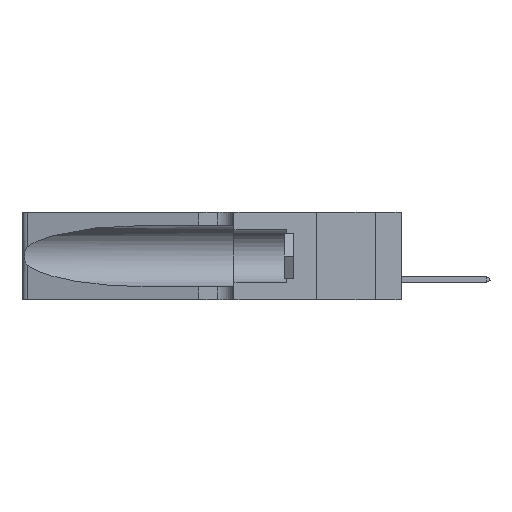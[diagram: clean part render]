
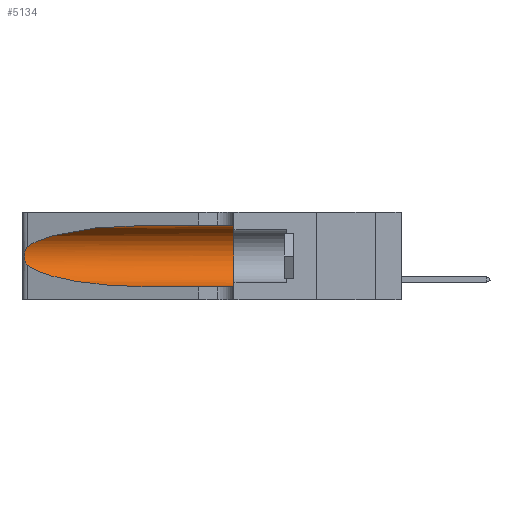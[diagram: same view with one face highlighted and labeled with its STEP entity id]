
A CAD part, left-side view. The second image highlights one B-rep face of the part: STEP entity #5134.
In plain terms, the highlighted cylindrical face has radius 3.308 mm (diameter 6.617 mm), a partial arc.
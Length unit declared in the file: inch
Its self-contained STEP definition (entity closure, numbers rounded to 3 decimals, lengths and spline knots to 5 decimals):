
#425 = AXIS2_PLACEMENT_3D ( 'NONE', #13948, #22495, #15842 ) ;
#451 = CARTESIAN_POINT ( 'NONE',  ( 0.25555, 1.22993, 0.14849 ) ) ;
#1627 = CARTESIAN_POINT ( 'NONE',  ( 0.25487, 1.22718, 0.22369 ) ) ;
#2332 = EDGE_CURVE ( 'NONE', #14540, #21522, #24726, .T. ) ;
#2381 =( BOUNDED_CURVE ( )  B_SPLINE_CURVE ( 3, ( #17505, #17337, #19689, #6827 ),
 .UNSPECIFIED., .F., .F. ) 
 B_SPLINE_CURVE_WITH_KNOTS ( ( 4, 4 ),
 ( 3.44316, 4.71239 ),
 .UNSPECIFIED. ) 
 CURVE ( )  GEOMETRIC_REPRESENTATION_ITEM ( )  RATIONAL_B_SPLINE_CURVE ( ( 1., 0.87, 0.87, 1. ) ) 
 REPRESENTATION_ITEM ( '' )  );
#2425 = ORIENTED_EDGE ( 'NONE', *, *, #22101, .T. ) ;
#2613 = CARTESIAN_POINT ( 'NONE',  ( 0.25639, 1.23184, 0.21858 ) ) ;
#3595 = CARTESIAN_POINT ( 'NONE',  ( 0.1305, 0.35, 0.185 ) ) ;
#4164 = CYLINDRICAL_SURFACE ( 'NONE', #425, 0.13025 ) ;
#4489 = VECTOR ( 'NONE', #23959, 39.37008 ) ;
#5134 = ADVANCED_FACE ( 'NONE', ( #15880 ), #4164, .F. ) ;
#5215 = ORIENTED_EDGE ( 'NONE', *, *, #2332, .T. ) ;
#6329 = VERTEX_POINT ( 'NONE', #11750 ) ;
#6827 = CARTESIAN_POINT ( 'NONE',  ( 0.1305, 0.72297, 0.05475 ) ) ;
#6933 = CARTESIAN_POINT ( 'NONE',  ( 0.25856, 1.23593, 0.16098 ) ) ;
#7114 = CARTESIAN_POINT ( 'NONE',  ( 0.25787, 1.23484, 0.2124 ) ) ;
#8302 = VECTOR ( 'NONE', #26611, 39.37008 ) ;
#8543 = CARTESIAN_POINT ( 'NONE',  ( 0.1305, 0.35, 0.05475 ) ) ;
#8867 = CARTESIAN_POINT ( 'NONE',  ( 0.25487, 1.22718, 0.14631 ) ) ;
#8982 = CARTESIAN_POINT ( 'NONE',  ( 0.1305, 1.61858, 0.31525 ) ) ;
#9100 = CARTESIAN_POINT ( 'NONE',  ( 0.25854, 1.2359, 0.20912 ) ) ;
#9189 = CARTESIAN_POINT ( 'NONE',  ( 0.26017, 1.23833, 0.17102 ) ) ;
#9274 = CARTESIAN_POINT ( 'NONE',  ( 0.26075, 1.23896, 0.19203 ) ) ;
#9334 = CIRCLE ( 'NONE', #10547, 0.13025 ) ;
#9367 = CARTESIAN_POINT ( 'NONE',  ( 0.25487, 1.22718, 0.14631 ) ) ;
#10216 = LINE ( 'NONE', #8982, #4489 ) ;
#10547 = AXIS2_PLACEMENT_3D ( 'NONE', #3595, #18323, #18415 ) ;
#11061 = VERTEX_POINT ( 'NONE', #17510 ) ;
#11353 = CARTESIAN_POINT ( 'NONE',  ( 0.25789, 1.23486, 0.15765 ) ) ;
#11530 = CARTESIAN_POINT ( 'NONE',  ( 0.26018, 1.23835, 0.19895 ) ) ;
#11750 = CARTESIAN_POINT ( 'NONE',  ( 0.1305, 0.72297, 0.31525 ) ) ;
#12284 = EDGE_CURVE ( 'NONE', #6329, #11061, #10216, .T. ) ;
#13278 = CARTESIAN_POINT ( 'NONE',  ( 0.1305, 0.72297, 0.05475 ) ) ;
#13948 = CARTESIAN_POINT ( 'NONE',  ( 0.1305, 1.61858, 0.185 ) ) ;
#14540 = VERTEX_POINT ( 'NONE', #1627 ) ;
#15487 = ORIENTED_EDGE ( 'NONE', *, *, #22920, .F. ) ;
#15822 = EDGE_CURVE ( 'NONE', #24346, #16372, #26017, .T. ) ;
#15842 = DIRECTION ( 'NONE',  ( 0., 0., -1. ) ) ;
#15880 = FACE_OUTER_BOUND ( 'NONE', #16827, .T. ) ;
#16372 = VERTEX_POINT ( 'NONE', #8543 ) ;
#16573 = ORIENTED_EDGE ( 'NONE', *, *, #20799, .T. ) ;
#16827 = EDGE_LOOP ( 'NONE', ( #2425, #5215, #16573, #27526, #15487, #18803 ) ) ;
#17337 = CARTESIAN_POINT ( 'NONE',  ( 0.2373, 1.15595, 0.08982 ) ) ;
#17505 = CARTESIAN_POINT ( 'NONE',  ( 0.25487, 1.22718, 0.14631 ) ) ;
#17510 = CARTESIAN_POINT ( 'NONE',  ( 0.1305, 0.35, 0.31525 ) ) ;
#17641 = CARTESIAN_POINT ( 'NONE',  ( 0.18966, 0.96281, 0.31525 ) ) ;
#17899 = CARTESIAN_POINT ( 'NONE',  ( 0.25555, 1.22994, 0.2215 ) ) ;
#18323 = DIRECTION ( 'NONE',  ( 0., 1., 0. ) ) ;
#18415 = DIRECTION ( 'NONE',  ( 0., 0., 1. ) ) ;
#18803 = ORIENTED_EDGE ( 'NONE', *, *, #12284, .F. ) ;
#19689 = CARTESIAN_POINT ( 'NONE',  ( 0.18966, 0.96281, 0.05475 ) ) ;
#19703 = CARTESIAN_POINT ( 'NONE',  ( 0.25639, 1.23186, 0.15144 ) ) ;
#19816 = CARTESIAN_POINT ( 'NONE',  ( 0.2373, 1.15595, 0.28018 ) ) ;
#19904 = CARTESIAN_POINT ( 'NONE',  ( 0.25487, 1.22718, 0.22369 ) ) ;
#20287 =( BOUNDED_CURVE ( )  B_SPLINE_CURVE ( 3, ( #26120, #17641, #19816, #19904 ),
 .UNSPECIFIED., .F., .T. ) 
 B_SPLINE_CURVE_WITH_KNOTS ( ( 4, 4 ),
 ( 1.5708, 2.84003 ),
 .UNSPECIFIED. ) 
 CURVE ( )  GEOMETRIC_REPRESENTATION_ITEM ( )  RATIONAL_B_SPLINE_CURVE ( ( 1., 0.87, 0.87, 1. ) ) 
 REPRESENTATION_ITEM ( '' )  );
#20799 = EDGE_CURVE ( 'NONE', #21522, #24346, #2381, .T. ) ;
#21522 = VERTEX_POINT ( 'NONE', #8867 ) ;
#22036 = CARTESIAN_POINT ( 'NONE',  ( 0.25487, 1.22718, 0.22369 ) ) ;
#22101 = EDGE_CURVE ( 'NONE', #6329, #14540, #20287, .T. ) ;
#22463 = CARTESIAN_POINT ( 'NONE',  ( 0.1305, 1.61858, 0.05475 ) ) ;
#22495 = DIRECTION ( 'NONE',  ( 0., -1., 0. ) ) ;
#22920 = EDGE_CURVE ( 'NONE', #11061, #16372, #9334, .T. ) ;
#23959 = DIRECTION ( 'NONE',  ( 0., -1., 0. ) ) ;
#24346 = VERTEX_POINT ( 'NONE', #13278 ) ;
#24726 = B_SPLINE_CURVE_WITH_KNOTS ( 'NONE', 3,
 ( #22036, #17899, #2613, #7114, #9100, #11530, #9274, #26200, #9189, #6933, #11353, #19703, #451, #9367 ),
 .UNSPECIFIED., .F., .F.,
 ( 4, 2, 2, 2, 2, 2, 4 ),
 ( 0., 0.00027, 0.00053, 0.00107, 0.0016, 0.00187, 0.00214 ),
 .UNSPECIFIED. ) ;
#26017 = LINE ( 'NONE', #22463, #8302 ) ;
#26120 = CARTESIAN_POINT ( 'NONE',  ( 0.1305, 0.72297, 0.31525 ) ) ;
#26200 = CARTESIAN_POINT ( 'NONE',  ( 0.26075, 1.23896, 0.178 ) ) ;
#26611 = DIRECTION ( 'NONE',  ( 0., -1., 0. ) ) ;
#27526 = ORIENTED_EDGE ( 'NONE', *, *, #15822, .T. ) ;
